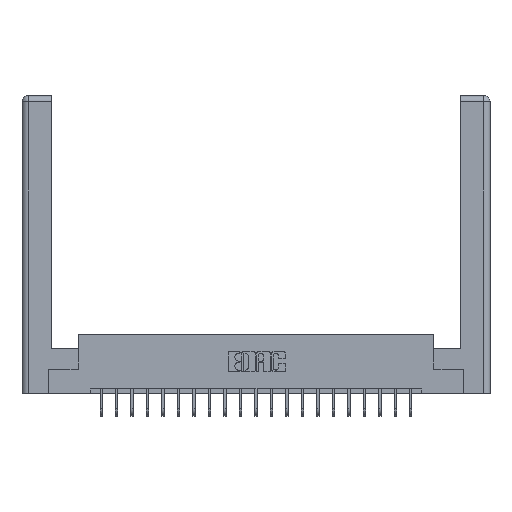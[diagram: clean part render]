
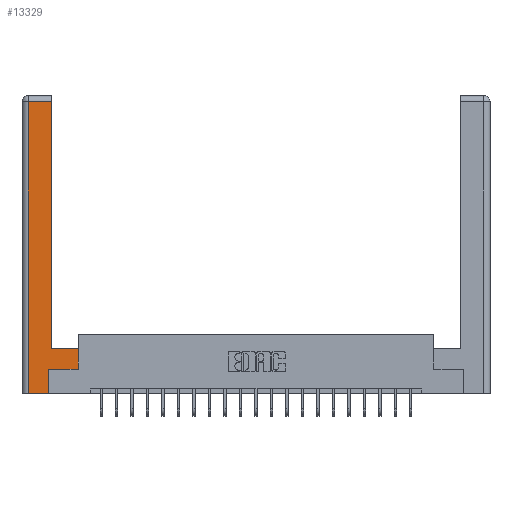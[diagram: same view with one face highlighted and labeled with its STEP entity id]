
A CAD part, top view. The second image highlights one B-rep face of the part: STEP entity #13329.
In plain terms, the highlighted planar face has unit normal (0, 0, 1).
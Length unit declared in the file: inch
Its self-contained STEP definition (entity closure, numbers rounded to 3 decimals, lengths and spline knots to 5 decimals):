
#8 = PLANE ( 'NONE',  #1959 ) ;
#1814 = EDGE_CURVE ( 'NONE', #8033, #2808, #23302, .T. ) ;
#1959 = AXIS2_PLACEMENT_3D ( 'NONE', #10887, #12774, #18263 ) ;
#2330 = EDGE_CURVE ( 'NONE', #14381, #8012, #20735, .T. ) ;
#2649 = LINE ( 'NONE', #21185, #6308 ) ;
#2808 = VERTEX_POINT ( 'NONE', #9883 ) ;
#3729 = CARTESIAN_POINT ( 'NONE',  ( 0.565, 0.245, 0. ) ) ;
#3773 = CARTESIAN_POINT ( 'NONE',  ( 0.295, 0.45, 0. ) ) ;
#3782 = CARTESIAN_POINT ( 'NONE',  ( 0.0615, 2.94, 0. ) ) ;
#4155 = CARTESIAN_POINT ( 'NONE',  ( 0.265, 0.245, 0. ) ) ;
#5098 = ORIENTED_EDGE ( 'NONE', *, *, #5963, .T. ) ;
#5742 = DIRECTION ( 'NONE',  ( -1., 0., 0. ) ) ;
#5963 = EDGE_CURVE ( 'NONE', #2808, #6666, #15448, .T. ) ;
#6194 = FACE_OUTER_BOUND ( 'NONE', #18213, .T. ) ;
#6203 = EDGE_CURVE ( 'NONE', #19661, #19018, #2649, .T. ) ;
#6308 = VECTOR ( 'NONE', #19284, 39.37008 ) ;
#6666 = VERTEX_POINT ( 'NONE', #18208 ) ;
#6780 = CARTESIAN_POINT ( 'NONE',  ( 0.295, 0.45, 0. ) ) ;
#7375 = CARTESIAN_POINT ( 'NONE',  ( 0.0615, 2.94, 0. ) ) ;
#7475 = DIRECTION ( 'NONE',  ( 1., 0., 0. ) ) ;
#8012 = VERTEX_POINT ( 'NONE', #7375 ) ;
#8033 = VERTEX_POINT ( 'NONE', #4155 ) ;
#8639 = DIRECTION ( 'NONE',  ( 0., -1., 0. ) ) ;
#8704 = ORIENTED_EDGE ( 'NONE', *, *, #11075, .T. ) ;
#9103 = VECTOR ( 'NONE', #16211, 39.37008 ) ;
#9566 = ORIENTED_EDGE ( 'NONE', *, *, #6203, .T. ) ;
#9826 = VECTOR ( 'NONE', #14867, 39.37008 ) ;
#9883 = CARTESIAN_POINT ( 'NONE',  ( 0.565, 0.245, 0. ) ) ;
#9990 = LINE ( 'NONE', #14534, #18512 ) ;
#10887 = CARTESIAN_POINT ( 'NONE',  ( 0., 0., 0. ) ) ;
#11075 = EDGE_CURVE ( 'NONE', #13304, #14381, #9990, .T. ) ;
#11281 = ORIENTED_EDGE ( 'NONE', *, *, #21278, .T. ) ;
#11895 = ORIENTED_EDGE ( 'NONE', *, *, #1814, .T. ) ;
#12774 = DIRECTION ( 'NONE',  ( 0., 0., -1. ) ) ;
#13304 = VERTEX_POINT ( 'NONE', #6780 ) ;
#13329 = ADVANCED_FACE ( 'NONE', ( #6194 ), #8, .F. ) ;
#13410 = CARTESIAN_POINT ( 'NONE',  ( 0.295, 2.94, 0. ) ) ;
#13978 = CARTESIAN_POINT ( 'NONE',  ( 0.565, 0.45, 0. ) ) ;
#14277 = CARTESIAN_POINT ( 'NONE',  ( 0.0615, 0., 0. ) ) ;
#14281 = EDGE_CURVE ( 'NONE', #19018, #8033, #23446, .T. ) ;
#14381 = VERTEX_POINT ( 'NONE', #13410 ) ;
#14534 = CARTESIAN_POINT ( 'NONE',  ( 0.295, 3., 0. ) ) ;
#14795 = VECTOR ( 'NONE', #7475, 39.37008 ) ;
#14867 = DIRECTION ( 'NONE',  ( 0., 1., 0. ) ) ;
#15448 = LINE ( 'NONE', #13978, #20855 ) ;
#15630 = DIRECTION ( 'NONE',  ( 0., 1., 0. ) ) ;
#16211 = DIRECTION ( 'NONE',  ( -1., 0., 0. ) ) ;
#16602 = CARTESIAN_POINT ( 'NONE',  ( 0.265, 0.245, 0. ) ) ;
#16957 = LINE ( 'NONE', #3773, #17533 ) ;
#17509 = LINE ( 'NONE', #14277, #20927 ) ;
#17533 = VECTOR ( 'NONE', #5742, 39.37008 ) ;
#18208 = CARTESIAN_POINT ( 'NONE',  ( 0.565, 0.45, 0. ) ) ;
#18213 = EDGE_LOOP ( 'NONE', ( #8704, #20249, #11281, #9566, #22079, #11895, #5098, #22847 ) ) ;
#18263 = DIRECTION ( 'NONE',  ( -1., 0., 0. ) ) ;
#18274 = CARTESIAN_POINT ( 'NONE',  ( 0.0615, 0., 0. ) ) ;
#18512 = VECTOR ( 'NONE', #19918, 39.37008 ) ;
#19018 = VERTEX_POINT ( 'NONE', #22022 ) ;
#19284 = DIRECTION ( 'NONE',  ( 1., 0., 0. ) ) ;
#19661 = VERTEX_POINT ( 'NONE', #18274 ) ;
#19918 = DIRECTION ( 'NONE',  ( 0., 1., 0. ) ) ;
#20249 = ORIENTED_EDGE ( 'NONE', *, *, #2330, .T. ) ;
#20735 = LINE ( 'NONE', #3782, #9103 ) ;
#20844 = EDGE_CURVE ( 'NONE', #6666, #13304, #16957, .T. ) ;
#20855 = VECTOR ( 'NONE', #15630, 39.37008 ) ;
#20927 = VECTOR ( 'NONE', #8639, 39.37008 ) ;
#21185 = CARTESIAN_POINT ( 'NONE',  ( 0.265, 0., 0. ) ) ;
#21278 = EDGE_CURVE ( 'NONE', #8012, #19661, #17509, .T. ) ;
#22022 = CARTESIAN_POINT ( 'NONE',  ( 0.265, 0., 0. ) ) ;
#22079 = ORIENTED_EDGE ( 'NONE', *, *, #14281, .T. ) ;
#22847 = ORIENTED_EDGE ( 'NONE', *, *, #20844, .T. ) ;
#23302 = LINE ( 'NONE', #3729, #14795 ) ;
#23446 = LINE ( 'NONE', #16602, #9826 ) ;
